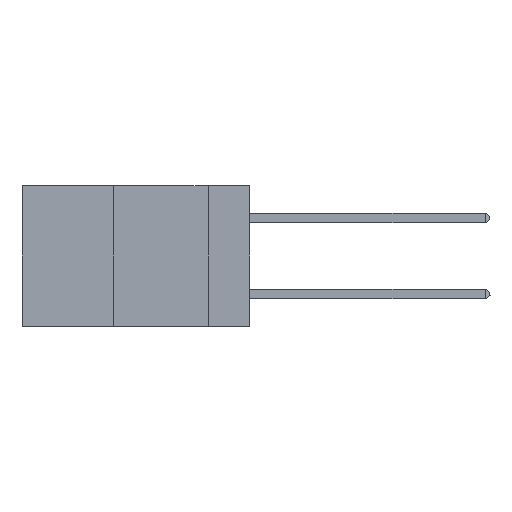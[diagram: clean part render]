
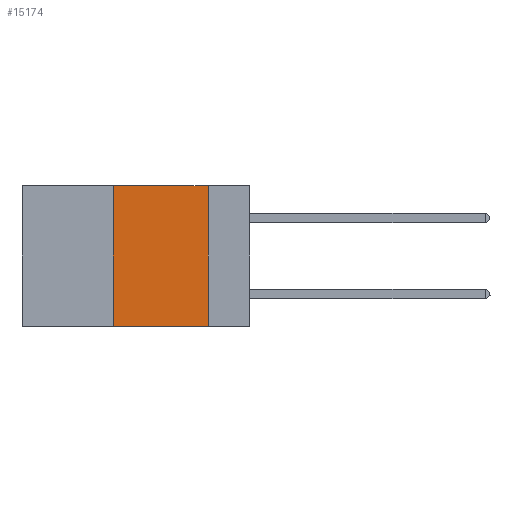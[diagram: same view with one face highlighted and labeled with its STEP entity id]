
A CAD part, left-side view. The second image highlights one B-rep face of the part: STEP entity #15174.
In plain terms, the highlighted planar face has unit normal (-1, 0, 0).
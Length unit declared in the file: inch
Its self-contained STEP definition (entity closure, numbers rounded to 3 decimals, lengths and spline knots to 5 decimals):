
#607 = EDGE_CURVE ( 'NONE', #3326, #10671, #16860, .T. ) ;
#1139 = CARTESIAN_POINT ( 'NONE',  ( 0., 0.36, -0.37 ) ) ;
#1905 = CARTESIAN_POINT ( 'NONE',  ( 0., 0.6, 0. ) ) ;
#2308 = EDGE_CURVE ( 'NONE', #12292, #3326, #11421, .T. ) ;
#3023 = DIRECTION ( 'NONE',  ( 0., -1., 0. ) ) ;
#3326 = VERTEX_POINT ( 'NONE', #8701 ) ;
#5079 = CARTESIAN_POINT ( 'NONE',  ( 0., 0.6, 0. ) ) ;
#5815 = ORIENTED_EDGE ( 'NONE', *, *, #11803, .F. ) ;
#6188 = VECTOR ( 'NONE', #3023, 39.37008 ) ;
#6634 = CARTESIAN_POINT ( 'NONE',  ( 0., 0.36, 0. ) ) ;
#6712 = ORIENTED_EDGE ( 'NONE', *, *, #8280, .T. ) ;
#7238 = ORIENTED_EDGE ( 'NONE', *, *, #2308, .F. ) ;
#7802 = PLANE ( 'NONE',  #14697 ) ;
#8280 = EDGE_CURVE ( 'NONE', #10137, #10671, #16542, .T. ) ;
#8399 = CARTESIAN_POINT ( 'NONE',  ( 0., 0.11, 0. ) ) ;
#8701 = CARTESIAN_POINT ( 'NONE',  ( 0., 0.11, 0. ) ) ;
#9710 = VECTOR ( 'NONE', #13667, 39.37008 ) ;
#9990 = DIRECTION ( 'NONE',  ( 0., -1., 0. ) ) ;
#10137 = VERTEX_POINT ( 'NONE', #1139 ) ;
#10332 = LINE ( 'NONE', #6634, #12219 ) ;
#10671 = VERTEX_POINT ( 'NONE', #16072 ) ;
#10785 = DIRECTION ( 'NONE',  ( 0., 0., 1. ) ) ;
#11351 = CARTESIAN_POINT ( 'NONE',  ( 0., 0.6, -0.37 ) ) ;
#11421 = LINE ( 'NONE', #1905, #6188 ) ;
#11749 = VECTOR ( 'NONE', #9990, 39.37008 ) ;
#11803 = EDGE_CURVE ( 'NONE', #10137, #12292, #10332, .T. ) ;
#11944 = CARTESIAN_POINT ( 'NONE',  ( 0., 0.36, 0. ) ) ;
#12219 = VECTOR ( 'NONE', #10785, 39.37008 ) ;
#12292 = VERTEX_POINT ( 'NONE', #11944 ) ;
#12664 = FACE_OUTER_BOUND ( 'NONE', #13591, .T. ) ;
#13233 = DIRECTION ( 'NONE',  ( 1., 0., 0. ) ) ;
#13591 = EDGE_LOOP ( 'NONE', ( #14788, #7238, #5815, #6712 ) ) ;
#13667 = DIRECTION ( 'NONE',  ( 0., 0., -1. ) ) ;
#14697 = AXIS2_PLACEMENT_3D ( 'NONE', #5079, #13233, #15917 ) ;
#14788 = ORIENTED_EDGE ( 'NONE', *, *, #607, .F. ) ;
#15174 = ADVANCED_FACE ( 'NONE', ( #12664 ), #7802, .F. ) ;
#15917 = DIRECTION ( 'NONE',  ( 0., 0., -1. ) ) ;
#16072 = CARTESIAN_POINT ( 'NONE',  ( 0., 0.11, -0.37 ) ) ;
#16542 = LINE ( 'NONE', #11351, #11749 ) ;
#16860 = LINE ( 'NONE', #8399, #9710 ) ;
